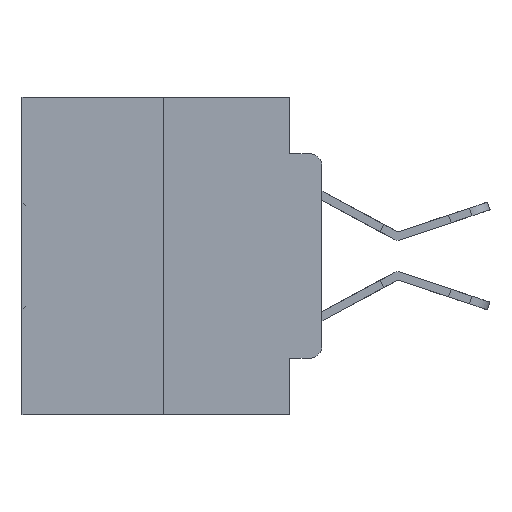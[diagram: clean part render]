
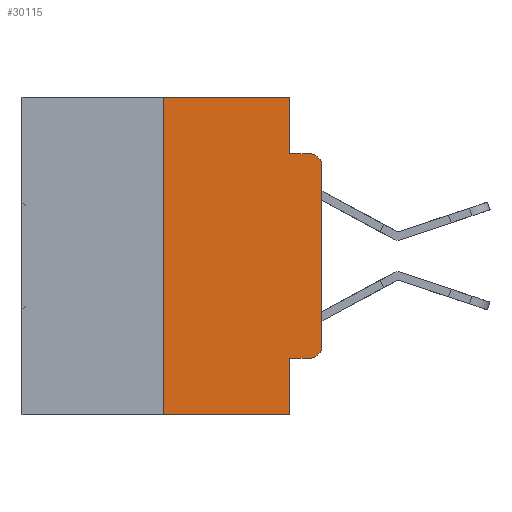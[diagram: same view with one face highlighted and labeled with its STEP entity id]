
A CAD part, left-side view. The second image highlights one B-rep face of the part: STEP entity #30115.
In plain terms, the highlighted planar face has unit normal (-1, 0, 0).
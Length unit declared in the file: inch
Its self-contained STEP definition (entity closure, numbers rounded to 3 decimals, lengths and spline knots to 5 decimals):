
#686 = VERTEX_POINT ( 'NONE', #20047 ) ;
#713 = ORIENTED_EDGE ( 'NONE', *, *, #18207, .F. ) ;
#948 = ORIENTED_EDGE ( 'NONE', *, *, #14940, .F. ) ;
#1043 = ORIENTED_EDGE ( 'NONE', *, *, #28760, .T. ) ;
#1210 = DIRECTION ( 'NONE',  ( 0., 0., -1. ) ) ;
#1868 = DIRECTION ( 'NONE',  ( 0., 0., -1. ) ) ;
#1881 = CIRCLE ( 'NONE', #23238, 0.02 ) ;
#2181 = VERTEX_POINT ( 'NONE', #17386 ) ;
#3459 = ORIENTED_EDGE ( 'NONE', *, *, #19517, .T. ) ;
#3844 = VECTOR ( 'NONE', #14556, 39.37008 ) ;
#3890 = PLANE ( 'NONE',  #20746 ) ;
#4271 = ORIENTED_EDGE ( 'NONE', *, *, #14470, .T. ) ;
#4282 = VECTOR ( 'NONE', #29128, 39.37008 ) ;
#5902 = DIRECTION ( 'NONE',  ( 0., 0., 1. ) ) ;
#6003 = EDGE_CURVE ( 'NONE', #21695, #686, #28878, .T. ) ;
#6230 = CARTESIAN_POINT ( 'NONE',  ( 0., 0.25, 0. ) ) ;
#6394 = VERTEX_POINT ( 'NONE', #27879 ) ;
#6982 = EDGE_LOOP ( 'NONE', ( #23434, #1043, #713, #13932, #20140, #7503, #4271, #948, #20591, #3459 ) ) ;
#7078 = CARTESIAN_POINT ( 'NONE',  ( 0., 0., -0.3915 ) ) ;
#7433 = LINE ( 'NONE', #30051, #20182 ) ;
#7503 = ORIENTED_EDGE ( 'NONE', *, *, #9143, .F. ) ;
#7540 = CARTESIAN_POINT ( 'NONE',  ( 0., 0., -0.1085 ) ) ;
#7705 = VECTOR ( 'NONE', #30614, 39.37008 ) ;
#7729 = VERTEX_POINT ( 'NONE', #7540 ) ;
#8365 = DIRECTION ( 'NONE',  ( 0., -1., 0. ) ) ;
#8650 = EDGE_CURVE ( 'NONE', #9203, #9939, #32610, .T. ) ;
#8953 = CIRCLE ( 'NONE', #30709, 0.02 ) ;
#9016 = CARTESIAN_POINT ( 'NONE',  ( 0., 0.051, -0.5 ) ) ;
#9018 = CARTESIAN_POINT ( 'NONE',  ( 0., 0.473, 0. ) ) ;
#9143 = EDGE_CURVE ( 'NONE', #2181, #9203, #31471, .T. ) ;
#9153 = DIRECTION ( 'NONE',  ( -1., 0., 0. ) ) ;
#9203 = VERTEX_POINT ( 'NONE', #6230 ) ;
#9697 = DIRECTION ( 'NONE',  ( 0., 0., -1. ) ) ;
#9939 = VERTEX_POINT ( 'NONE', #22584 ) ;
#11526 = DIRECTION ( 'NONE',  ( 0., 0., -1. ) ) ;
#11808 = LINE ( 'NONE', #31655, #4282 ) ;
#13932 = ORIENTED_EDGE ( 'NONE', *, *, #29551, .F. ) ;
#14320 = VERTEX_POINT ( 'NONE', #9016 ) ;
#14470 = EDGE_CURVE ( 'NONE', #2181, #14320, #30898, .T. ) ;
#14556 = DIRECTION ( 'NONE',  ( 0., -1., 0. ) ) ;
#14940 = EDGE_CURVE ( 'NONE', #21695, #14320, #24183, .T. ) ;
#15843 = FACE_OUTER_BOUND ( 'NONE', #6982, .T. ) ;
#16059 = CARTESIAN_POINT ( 'NONE',  ( 0., 0.25, 0. ) ) ;
#16576 = VECTOR ( 'NONE', #1210, 39.37008 ) ;
#16999 = CARTESIAN_POINT ( 'NONE',  ( 0., 0.02, -0.0885 ) ) ;
#17128 = DIRECTION ( 'NONE',  ( -1., 0., 0. ) ) ;
#17149 = CARTESIAN_POINT ( 'NONE',  ( 0., 0.473, -0.5 ) ) ;
#17386 = CARTESIAN_POINT ( 'NONE',  ( 0., 0.25, -0.5 ) ) ;
#18207 = EDGE_CURVE ( 'NONE', #6394, #18940, #11808, .T. ) ;
#18940 = VERTEX_POINT ( 'NONE', #16999 ) ;
#19010 = CARTESIAN_POINT ( 'NONE',  ( 0., 0.051, 0. ) ) ;
#19390 = CARTESIAN_POINT ( 'NONE',  ( 0., 0.051, -0.4115 ) ) ;
#19517 = EDGE_CURVE ( 'NONE', #686, #22932, #1881, .T. ) ;
#20047 = CARTESIAN_POINT ( 'NONE',  ( 0., 0.02, -0.4115 ) ) ;
#20140 = ORIENTED_EDGE ( 'NONE', *, *, #8650, .F. ) ;
#20182 = VECTOR ( 'NONE', #9697, 39.37008 ) ;
#20591 = ORIENTED_EDGE ( 'NONE', *, *, #6003, .T. ) ;
#20746 = AXIS2_PLACEMENT_3D ( 'NONE', #9018, #26823, #11526 ) ;
#21279 = EDGE_CURVE ( 'NONE', #22932, #7729, #28809, .T. ) ;
#21310 = DIRECTION ( 'NONE',  ( 0., -1., 0. ) ) ;
#21695 = VERTEX_POINT ( 'NONE', #19390 ) ;
#22143 = VECTOR ( 'NONE', #8365, 39.37008 ) ;
#22584 = CARTESIAN_POINT ( 'NONE',  ( 0., 0.051, 0. ) ) ;
#22932 = VERTEX_POINT ( 'NONE', #7078 ) ;
#23238 = AXIS2_PLACEMENT_3D ( 'NONE', #24448, #9153, #26975 ) ;
#23434 = ORIENTED_EDGE ( 'NONE', *, *, #21279, .T. ) ;
#23992 = VECTOR ( 'NONE', #5902, 39.37008 ) ;
#24183 = LINE ( 'NONE', #19010, #16576 ) ;
#24448 = CARTESIAN_POINT ( 'NONE',  ( 0., 0.02, -0.3915 ) ) ;
#26734 = VECTOR ( 'NONE', #21310, 39.37008 ) ;
#26823 = DIRECTION ( 'NONE',  ( 1., 0., 0. ) ) ;
#26975 = DIRECTION ( 'NONE',  ( 0., 0., -1. ) ) ;
#27879 = CARTESIAN_POINT ( 'NONE',  ( 0., 0.051, -0.0885 ) ) ;
#28077 = CARTESIAN_POINT ( 'NONE',  ( 0., 0., 0. ) ) ;
#28723 = CARTESIAN_POINT ( 'NONE',  ( 0., 0.051, -0.4115 ) ) ;
#28760 = EDGE_CURVE ( 'NONE', #7729, #18940, #8953, .T. ) ;
#28809 = LINE ( 'NONE', #28077, #7705 ) ;
#28878 = LINE ( 'NONE', #28723, #22143 ) ;
#29128 = DIRECTION ( 'NONE',  ( 0., -1., 0. ) ) ;
#29551 = EDGE_CURVE ( 'NONE', #9939, #6394, #7433, .T. ) ;
#30051 = CARTESIAN_POINT ( 'NONE',  ( 0., 0.051, 0. ) ) ;
#30115 = ADVANCED_FACE ( 'NONE', ( #15843 ), #3890, .F. ) ;
#30614 = DIRECTION ( 'NONE',  ( 0., 0., 1. ) ) ;
#30709 = AXIS2_PLACEMENT_3D ( 'NONE', #32275, #17128, #1868 ) ;
#30898 = LINE ( 'NONE', #17149, #3844 ) ;
#31387 = CARTESIAN_POINT ( 'NONE',  ( 0., 0.473, 0. ) ) ;
#31471 = LINE ( 'NONE', #16059, #23992 ) ;
#31655 = CARTESIAN_POINT ( 'NONE',  ( 0., 0.051, -0.0885 ) ) ;
#32275 = CARTESIAN_POINT ( 'NONE',  ( 0., 0.02, -0.1085 ) ) ;
#32610 = LINE ( 'NONE', #31387, #26734 ) ;
